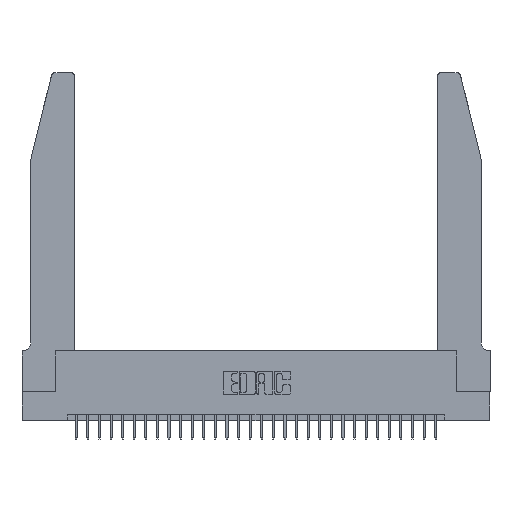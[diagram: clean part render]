
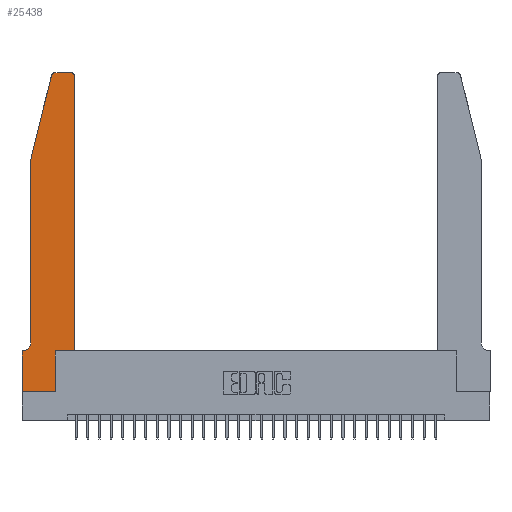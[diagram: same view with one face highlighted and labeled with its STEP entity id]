
A CAD part, top view. The second image highlights one B-rep face of the part: STEP entity #25438.
In plain terms, the highlighted planar face has unit normal (0, 0, 1).
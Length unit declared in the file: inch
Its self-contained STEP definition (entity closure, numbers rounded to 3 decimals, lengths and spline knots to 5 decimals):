
#446 = DIRECTION ( 'NONE',  ( 0., -1., 0. ) ) ;
#626 = VERTEX_POINT ( 'NONE', #12203 ) ;
#831 = ORIENTED_EDGE ( 'NONE', *, *, #7826, .T. ) ;
#1008 = DIRECTION ( 'NONE',  ( 1., 0., 0. ) ) ;
#1095 = EDGE_CURVE ( 'NONE', #17537, #21907, #20190, .T. ) ;
#1601 = EDGE_CURVE ( 'NONE', #24844, #626, #10590, .T. ) ;
#1975 = CIRCLE ( 'NONE', #6278, 0.07 ) ;
#3122 = VECTOR ( 'NONE', #17207, 39.37008 ) ;
#3475 = LINE ( 'NONE', #26583, #4997 ) ;
#3628 = VERTEX_POINT ( 'NONE', #7305 ) ;
#3700 = VERTEX_POINT ( 'NONE', #14593 ) ;
#3904 = CIRCLE ( 'NONE', #6469, 0.03 ) ;
#4179 = CARTESIAN_POINT ( 'NONE',  ( 0.4505, 0.35, 0.37 ) ) ;
#4997 = VECTOR ( 'NONE', #18995, 39.37008 ) ;
#5203 = DIRECTION ( 'NONE',  ( -1., 0., 0. ) ) ;
#5361 = VECTOR ( 'NONE', #446, 39.37008 ) ;
#5381 = ORIENTED_EDGE ( 'NONE', *, *, #20923, .T. ) ;
#5810 = CARTESIAN_POINT ( 'NONE',  ( 0.0755, 0.42, 0.37 ) ) ;
#5999 = VERTEX_POINT ( 'NONE', #29297 ) ;
#6209 = EDGE_CURVE ( 'NONE', #3628, #24844, #3904, .T. ) ;
#6278 = AXIS2_PLACEMENT_3D ( 'NONE', #26748, #19569, #19665 ) ;
#6290 = ORIENTED_EDGE ( 'NONE', *, *, #13498, .T. ) ;
#6373 = DIRECTION ( 'NONE',  ( 0., 1., 0. ) ) ;
#6407 = EDGE_CURVE ( 'NONE', #27126, #5999, #1975, .T. ) ;
#6469 = AXIS2_PLACEMENT_3D ( 'NONE', #7989, #20154, #1008 ) ;
#7305 = CARTESIAN_POINT ( 'NONE',  ( 0.4505, 2.72, 0.37 ) ) ;
#7333 = DIRECTION ( 'NONE',  ( 0., 1., 0. ) ) ;
#7423 = DIRECTION ( 'NONE',  ( -0.239, -0.971, 0. ) ) ;
#7499 = ORIENTED_EDGE ( 'NONE', *, *, #24477, .T. ) ;
#7519 = CARTESIAN_POINT ( 'NONE',  ( 0.0755, 2., 0.37 ) ) ;
#7623 = CARTESIAN_POINT ( 'NONE',  ( 0.0755, 2., 0.37 ) ) ;
#7826 = EDGE_CURVE ( 'NONE', #3700, #3628, #26874, .T. ) ;
#7989 = CARTESIAN_POINT ( 'NONE',  ( 0.4205, 2.72, 0.37 ) ) ;
#8048 = CARTESIAN_POINT ( 'NONE',  ( 0.4505, 0.35, 0.37 ) ) ;
#8955 = ORIENTED_EDGE ( 'NONE', *, *, #6407, .T. ) ;
#9141 = DIRECTION ( 'NONE',  ( 1., 0., 0. ) ) ;
#9556 = ORIENTED_EDGE ( 'NONE', *, *, #21089, .T. ) ;
#10590 = LINE ( 'NONE', #21473, #3122 ) ;
#10718 = CARTESIAN_POINT ( 'NONE',  ( 0.0755, 2., 0.37 ) ) ;
#11233 = CARTESIAN_POINT ( 'NONE',  ( 0., 0.35, 0.37 ) ) ;
#11325 = VECTOR ( 'NONE', #5203, 39.37008 ) ;
#11349 = VERTEX_POINT ( 'NONE', #15145 ) ;
#11507 = LINE ( 'NONE', #8048, #20174 ) ;
#11737 = DIRECTION ( 'NONE',  ( 0., 0., 1. ) ) ;
#11776 = CARTESIAN_POINT ( 'NONE',  ( 0.4205, 2.75, 0.37 ) ) ;
#11817 = LINE ( 'NONE', #7519, #5361 ) ;
#12203 = CARTESIAN_POINT ( 'NONE',  ( 0.284, 2.75, 0.37 ) ) ;
#12377 = CARTESIAN_POINT ( 'NONE',  ( 0.2865, 0., 0.37 ) ) ;
#13043 = DIRECTION ( 'NONE',  ( 1., 0., 0. ) ) ;
#13498 = EDGE_CURVE ( 'NONE', #21907, #13811, #3475, .T. ) ;
#13620 = EDGE_CURVE ( 'NONE', #29838, #27126, #11817, .T. ) ;
#13811 = VERTEX_POINT ( 'NONE', #12377 ) ;
#14167 = DIRECTION ( 'NONE',  ( 1., 0., 0. ) ) ;
#14593 = CARTESIAN_POINT ( 'NONE',  ( 0.4505, 0.35, 0.37 ) ) ;
#15145 = CARTESIAN_POINT ( 'NONE',  ( 0.25487, 2.72718, 0.37 ) ) ;
#16400 = CARTESIAN_POINT ( 'NONE',  ( 0., 0.35, 0.37 ) ) ;
#17207 = DIRECTION ( 'NONE',  ( -1., 0., 0. ) ) ;
#17367 = ORIENTED_EDGE ( 'NONE', *, *, #13620, .T. ) ;
#17506 = ORIENTED_EDGE ( 'NONE', *, *, #6209, .T. ) ;
#17537 = VERTEX_POINT ( 'NONE', #11233 ) ;
#17794 = ORIENTED_EDGE ( 'NONE', *, *, #28252, .T. ) ;
#18970 = DIRECTION ( 'NONE',  ( 0., 0., 1. ) ) ;
#18995 = DIRECTION ( 'NONE',  ( 1., 0., 0. ) ) ;
#19070 = AXIS2_PLACEMENT_3D ( 'NONE', #23611, #18970, #9141 ) ;
#19260 = LINE ( 'NONE', #24439, #11325 ) ;
#19455 = VECTOR ( 'NONE', #24369, 39.37008 ) ;
#19569 = DIRECTION ( 'NONE',  ( 0., 0., -1. ) ) ;
#19665 = DIRECTION ( 'NONE',  ( -1., 0., 0. ) ) ;
#19997 = VECTOR ( 'NONE', #7423, 39.37008 ) ;
#20154 = DIRECTION ( 'NONE',  ( 0., 0., 1. ) ) ;
#20174 = VECTOR ( 'NONE', #13043, 39.37008 ) ;
#20190 = LINE ( 'NONE', #21920, #19455 ) ;
#20422 = VECTOR ( 'NONE', #6373, 39.37008 ) ;
#20442 = FACE_OUTER_BOUND ( 'NONE', #30560, .T. ) ;
#20923 = EDGE_CURVE ( 'NONE', #11349, #29838, #29074, .T. ) ;
#21089 = EDGE_CURVE ( 'NONE', #25423, #3700, #11507, .T. ) ;
#21473 = CARTESIAN_POINT ( 'NONE',  ( 0.2605, 2.75, 0.37 ) ) ;
#21907 = VERTEX_POINT ( 'NONE', #31049 ) ;
#21920 = CARTESIAN_POINT ( 'NONE',  ( 0., 0., 0.37 ) ) ;
#23611 = CARTESIAN_POINT ( 'NONE',  ( 0.284, 2.72, 0.37 ) ) ;
#24369 = DIRECTION ( 'NONE',  ( 0., -1., 0. ) ) ;
#24439 = CARTESIAN_POINT ( 'NONE',  ( 0.0755, 0.35, 0.37 ) ) ;
#24477 = EDGE_CURVE ( 'NONE', #13811, #25423, #29972, .T. ) ;
#24844 = VERTEX_POINT ( 'NONE', #11776 ) ;
#25423 = VERTEX_POINT ( 'NONE', #26010 ) ;
#25438 = ADVANCED_FACE ( 'NONE', ( #20442 ), #28453, .T. ) ;
#26010 = CARTESIAN_POINT ( 'NONE',  ( 0.2865, 0.35, 0.37 ) ) ;
#26512 = AXIS2_PLACEMENT_3D ( 'NONE', #16400, #11737, #14167 ) ;
#26583 = CARTESIAN_POINT ( 'NONE',  ( 0., 0., 0.37 ) ) ;
#26748 = CARTESIAN_POINT ( 'NONE',  ( 0.0055, 0.42, 0.37 ) ) ;
#26852 = ORIENTED_EDGE ( 'NONE', *, *, #1095, .T. ) ;
#26874 = LINE ( 'NONE', #4179, #20422 ) ;
#27126 = VERTEX_POINT ( 'NONE', #5810 ) ;
#27942 = EDGE_CURVE ( 'NONE', #5999, #17537, #19260, .T. ) ;
#28252 = EDGE_CURVE ( 'NONE', #626, #11349, #28386, .T. ) ;
#28386 = CIRCLE ( 'NONE', #19070, 0.03 ) ;
#28453 = PLANE ( 'NONE',  #26512 ) ;
#29074 = LINE ( 'NONE', #7623, #19997 ) ;
#29125 = CARTESIAN_POINT ( 'NONE',  ( 0.2865, 0.35, 0.37 ) ) ;
#29297 = CARTESIAN_POINT ( 'NONE',  ( 0.0055, 0.35, 0.37 ) ) ;
#29617 = VECTOR ( 'NONE', #7333, 39.37008 ) ;
#29647 = ORIENTED_EDGE ( 'NONE', *, *, #1601, .T. ) ;
#29838 = VERTEX_POINT ( 'NONE', #10718 ) ;
#29972 = LINE ( 'NONE', #29125, #29617 ) ;
#30510 = ORIENTED_EDGE ( 'NONE', *, *, #27942, .T. ) ;
#30560 = EDGE_LOOP ( 'NONE', ( #29647, #17794, #5381, #17367, #8955, #30510, #26852, #6290, #7499, #9556, #831, #17506 ) ) ;
#31049 = CARTESIAN_POINT ( 'NONE',  ( 0., 0., 0.37 ) ) ;
